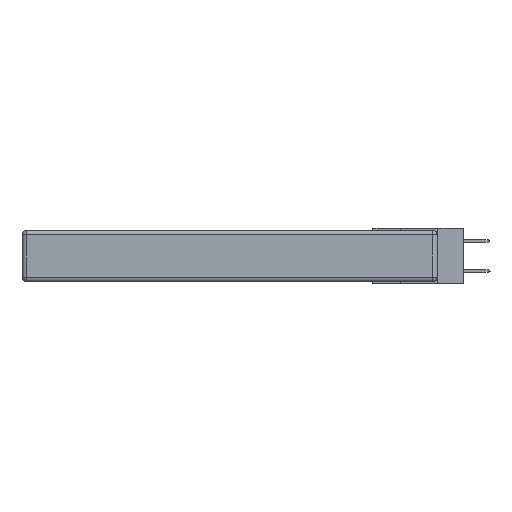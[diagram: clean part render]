
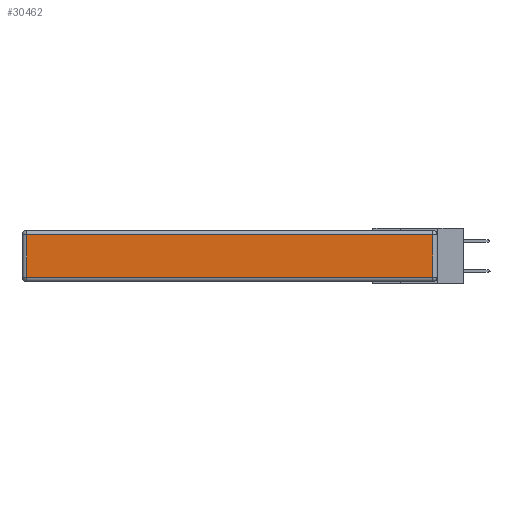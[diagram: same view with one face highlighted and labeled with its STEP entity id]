
A CAD part, left-side view. The second image highlights one B-rep face of the part: STEP entity #30462.
In plain terms, the highlighted planar face has unit normal (-1, 0, 0).
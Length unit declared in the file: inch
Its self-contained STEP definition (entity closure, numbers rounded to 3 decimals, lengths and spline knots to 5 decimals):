
#1407 = CARTESIAN_POINT ( 'NONE',  ( 0., 0., -0.313 ) ) ;
#2680 = DIRECTION ( 'NONE',  ( 0., 0., 1. ) ) ;
#2800 = PLANE ( 'NONE',  #9422 ) ;
#3024 = CARTESIAN_POINT ( 'NONE',  ( 0., 2.72, -0.343 ) ) ;
#3733 = ORIENTED_EDGE ( 'NONE', *, *, #29514, .T. ) ;
#5116 = CARTESIAN_POINT ( 'NONE',  ( 0., 0.03, -0.343 ) ) ;
#5216 = ORIENTED_EDGE ( 'NONE', *, *, #33850, .T. ) ;
#5723 = DIRECTION ( 'NONE',  ( 0., 0., -1. ) ) ;
#6399 = VERTEX_POINT ( 'NONE', #18065 ) ;
#6770 = DIRECTION ( 'NONE',  ( 0., 0., 1. ) ) ;
#6893 = CARTESIAN_POINT ( 'NONE',  ( 0., 2.75, -0.03 ) ) ;
#7280 = EDGE_CURVE ( 'NONE', #15565, #6399, #26253, .T. ) ;
#9088 = EDGE_CURVE ( 'NONE', #15394, #10125, #12098, .T. ) ;
#9422 = AXIS2_PLACEMENT_3D ( 'NONE', #16541, #19021, #2680 ) ;
#10125 = VERTEX_POINT ( 'NONE', #10662 ) ;
#10662 = CARTESIAN_POINT ( 'NONE',  ( 0., 0.03, -0.03 ) ) ;
#11072 = VECTOR ( 'NONE', #34987, 39.37008 ) ;
#11734 = FACE_OUTER_BOUND ( 'NONE', #19052, .T. ) ;
#12098 = LINE ( 'NONE', #5116, #26111 ) ;
#14025 = VECTOR ( 'NONE', #5723, 39.37008 ) ;
#14120 = LINE ( 'NONE', #1407, #11072 ) ;
#15394 = VERTEX_POINT ( 'NONE', #27538 ) ;
#15565 = VERTEX_POINT ( 'NONE', #31570 ) ;
#16541 = CARTESIAN_POINT ( 'NONE',  ( 0., 0., -0.343 ) ) ;
#18065 = CARTESIAN_POINT ( 'NONE',  ( 0., 2.72, -0.313 ) ) ;
#18489 = DIRECTION ( 'NONE',  ( 0., 1., 0. ) ) ;
#19021 = DIRECTION ( 'NONE',  ( -1., 0., 0. ) ) ;
#19052 = EDGE_LOOP ( 'NONE', ( #5216, #25910, #3733, #21246 ) ) ;
#21246 = ORIENTED_EDGE ( 'NONE', *, *, #7280, .T. ) ;
#23989 = LINE ( 'NONE', #6893, #30568 ) ;
#25910 = ORIENTED_EDGE ( 'NONE', *, *, #9088, .T. ) ;
#26111 = VECTOR ( 'NONE', #6770, 39.37008 ) ;
#26253 = LINE ( 'NONE', #3024, #14025 ) ;
#27538 = CARTESIAN_POINT ( 'NONE',  ( 0., 0.03, -0.313 ) ) ;
#29514 = EDGE_CURVE ( 'NONE', #10125, #15565, #23989, .T. ) ;
#30462 = ADVANCED_FACE ( 'NONE', ( #11734 ), #2800, .T. ) ;
#30568 = VECTOR ( 'NONE', #18489, 39.37008 ) ;
#31570 = CARTESIAN_POINT ( 'NONE',  ( 0., 2.72, -0.03 ) ) ;
#33850 = EDGE_CURVE ( 'NONE', #6399, #15394, #14120, .T. ) ;
#34987 = DIRECTION ( 'NONE',  ( 0., -1., 0. ) ) ;
